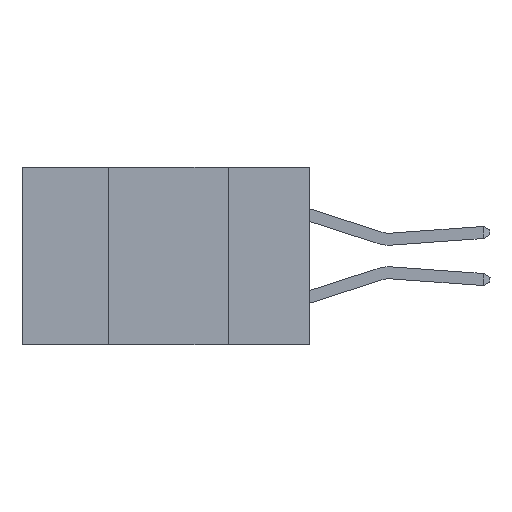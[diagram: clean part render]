
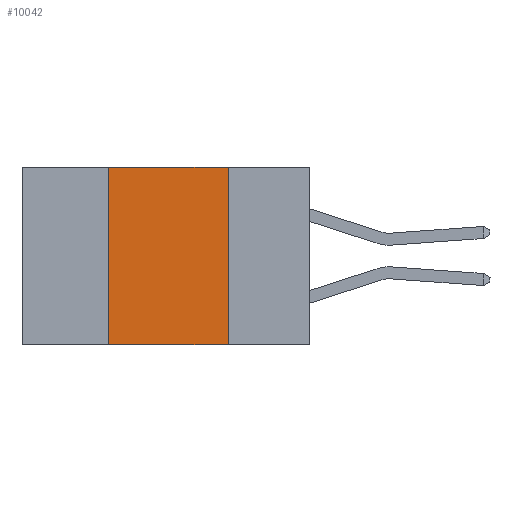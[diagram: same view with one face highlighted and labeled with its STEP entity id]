
A CAD part, left-side view. The second image highlights one B-rep face of the part: STEP entity #10042.
In plain terms, the highlighted planar face has unit normal (-1, 0, 0).
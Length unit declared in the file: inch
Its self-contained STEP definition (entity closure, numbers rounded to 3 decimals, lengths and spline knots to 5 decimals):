
#163 = VECTOR ( 'NONE', #17278, 39.37008 ) ;
#423 = EDGE_LOOP ( 'NONE', ( #8425, #15626, #12520, #16047 ) ) ;
#1519 = LINE ( 'NONE', #1730, #13593 ) ;
#1730 = CARTESIAN_POINT ( 'NONE',  ( 0., 0.17, -0.37 ) ) ;
#2082 = CARTESIAN_POINT ( 'NONE',  ( 0., 0.17, 0. ) ) ;
#2437 = CARTESIAN_POINT ( 'NONE',  ( 0., 0.17, -0.37 ) ) ;
#2847 = DIRECTION ( 'NONE',  ( 0., -1., 0. ) ) ;
#2866 = CARTESIAN_POINT ( 'NONE',  ( 0., 0.6, -0.37 ) ) ;
#3177 = DIRECTION ( 'NONE',  ( 1., 0., 0. ) ) ;
#4029 = EDGE_CURVE ( 'NONE', #6703, #15733, #7818, .T. ) ;
#4145 = LINE ( 'NONE', #15975, #163 ) ;
#4304 = VERTEX_POINT ( 'NONE', #6157 ) ;
#6157 = CARTESIAN_POINT ( 'NONE',  ( 0., 0.42, 0. ) ) ;
#6392 = VERTEX_POINT ( 'NONE', #2082 ) ;
#6703 = VERTEX_POINT ( 'NONE', #13679 ) ;
#7818 = LINE ( 'NONE', #2866, #11495 ) ;
#8425 = ORIENTED_EDGE ( 'NONE', *, *, #13709, .F. ) ;
#8807 = CARTESIAN_POINT ( 'NONE',  ( 0., 0.6, 0. ) ) ;
#10042 = ADVANCED_FACE ( 'NONE', ( #13723 ), #11570, .F. ) ;
#11360 = VECTOR ( 'NONE', #13788, 39.37008 ) ;
#11495 = VECTOR ( 'NONE', #2847, 39.37008 ) ;
#11570 = PLANE ( 'NONE',  #16242 ) ;
#11595 = DIRECTION ( 'NONE',  ( 0., 0., -1. ) ) ;
#12520 = ORIENTED_EDGE ( 'NONE', *, *, #16359, .F. ) ;
#12959 = DIRECTION ( 'NONE',  ( 0., 0., -1. ) ) ;
#13593 = VECTOR ( 'NONE', #11595, 39.37008 ) ;
#13679 = CARTESIAN_POINT ( 'NONE',  ( 0., 0.42, -0.37 ) ) ;
#13709 = EDGE_CURVE ( 'NONE', #6392, #15733, #1519, .T. ) ;
#13723 = FACE_OUTER_BOUND ( 'NONE', #423, .T. ) ;
#13788 = DIRECTION ( 'NONE',  ( 0., -1., 0. ) ) ;
#15626 = ORIENTED_EDGE ( 'NONE', *, *, #16634, .F. ) ;
#15733 = VERTEX_POINT ( 'NONE', #2437 ) ;
#15975 = CARTESIAN_POINT ( 'NONE',  ( 0., 0.42, -0.37 ) ) ;
#16047 = ORIENTED_EDGE ( 'NONE', *, *, #4029, .T. ) ;
#16242 = AXIS2_PLACEMENT_3D ( 'NONE', #8807, #3177, #12959 ) ;
#16359 = EDGE_CURVE ( 'NONE', #6703, #4304, #4145, .T. ) ;
#16634 = EDGE_CURVE ( 'NONE', #4304, #6392, #17984, .T. ) ;
#17278 = DIRECTION ( 'NONE',  ( 0., 0., 1. ) ) ;
#17730 = CARTESIAN_POINT ( 'NONE',  ( 0., 0.6, 0. ) ) ;
#17984 = LINE ( 'NONE', #17730, #11360 ) ;
